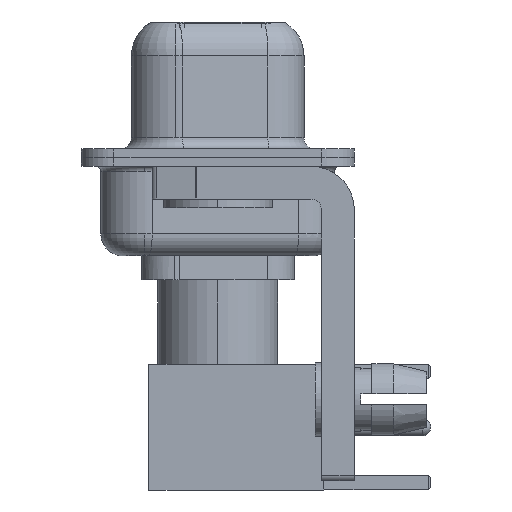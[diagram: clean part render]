
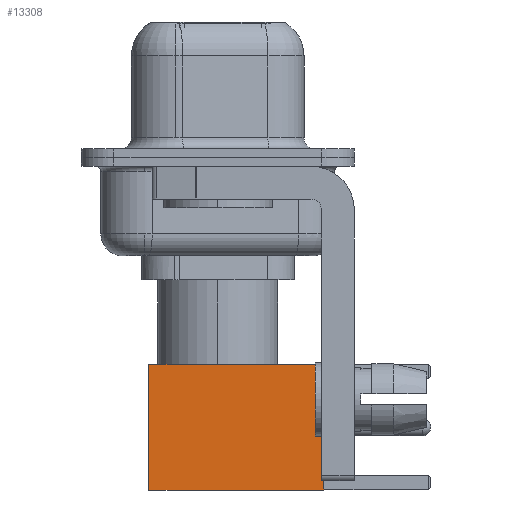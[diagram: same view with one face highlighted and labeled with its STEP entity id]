
A CAD part, left-side view. The second image highlights one B-rep face of the part: STEP entity #13308.
In plain terms, the highlighted face is planar.
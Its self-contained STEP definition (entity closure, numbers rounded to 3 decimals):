
#153 = DIRECTION ( 'NONE',  ( 0., 0., -1. ) ) ;
#1146 = VERTEX_POINT ( 'NONE', #7245 ) ;
#3455 = CARTESIAN_POINT ( 'NONE',  ( 0., 2.875, 8. ) ) ;
#3643 = DIRECTION ( 'NONE',  ( -1., 0., 0. ) ) ;
#3648 = CARTESIAN_POINT ( 'NONE',  ( 2.875, 2.875, 0. ) ) ;
#4043 = DIRECTION ( 'NONE',  ( 0., 0., -1. ) ) ;
#4792 = CARTESIAN_POINT ( 'NONE',  ( 2.875, 2.875, 0. ) ) ;
#6378 = VECTOR ( 'NONE', #9879, 1000. ) ;
#6505 = PLANE ( 'NONE',  #20114 ) ;
#7245 = CARTESIAN_POINT ( 'NONE',  ( 2.875, 2.875, 0. ) ) ;
#8069 = VECTOR ( 'NONE', #3643, 1000. ) ;
#8305 = VERTEX_POINT ( 'NONE', #12807 ) ;
#8445 = EDGE_CURVE ( 'NONE', #8305, #14419, #11447, .T. ) ;
#9879 = DIRECTION ( 'NONE',  ( -1., 0., 0. ) ) ;
#10093 = EDGE_CURVE ( 'NONE', #8305, #1146, #12885, .T. ) ;
#10465 = EDGE_CURVE ( 'NONE', #14419, #15791, #13902, .T. ) ;
#10764 = CARTESIAN_POINT ( 'NONE',  ( -2.875, 2.875, 0. ) ) ;
#11069 = ORIENTED_EDGE ( 'NONE', *, *, #13387, .T. ) ;
#11240 = ORIENTED_EDGE ( 'NONE', *, *, #10093, .T. ) ;
#11447 = LINE ( 'NONE', #3455, #6378 ) ;
#11632 = LINE ( 'NONE', #17826, #8069 ) ;
#11688 = ORIENTED_EDGE ( 'NONE', *, *, #10465, .F. ) ;
#12420 = ORIENTED_EDGE ( 'NONE', *, *, #8445, .F. ) ;
#12807 = CARTESIAN_POINT ( 'NONE',  ( 2.875, 2.875, 8. ) ) ;
#12885 = LINE ( 'NONE', #4792, #14811 ) ;
#13140 = VECTOR ( 'NONE', #4043, 1000. ) ;
#13308 = ADVANCED_FACE ( 'NONE', ( #14471 ), #6505, .T. ) ;
#13387 = EDGE_CURVE ( 'NONE', #1146, #15791, #11632, .T. ) ;
#13902 = LINE ( 'NONE', #10764, #13140 ) ;
#14363 = EDGE_LOOP ( 'NONE', ( #11240, #11069, #11688, #12420 ) ) ;
#14419 = VERTEX_POINT ( 'NONE', #15476 ) ;
#14471 = FACE_OUTER_BOUND ( 'NONE', #14363, .T. ) ;
#14811 = VECTOR ( 'NONE', #153, 1000. ) ;
#15476 = CARTESIAN_POINT ( 'NONE',  ( -2.875, 2.875, 8. ) ) ;
#15791 = VERTEX_POINT ( 'NONE', #19486 ) ;
#16454 = DIRECTION ( 'NONE',  ( 0., 0., 1. ) ) ;
#17826 = CARTESIAN_POINT ( 'NONE',  ( 0., 2.875, 0. ) ) ;
#19486 = CARTESIAN_POINT ( 'NONE',  ( -2.875, 2.875, 0. ) ) ;
#19616 = DIRECTION ( 'NONE',  ( 0., 1., 0. ) ) ;
#20114 = AXIS2_PLACEMENT_3D ( 'NONE', #3648, #19616, #16454 ) ;
